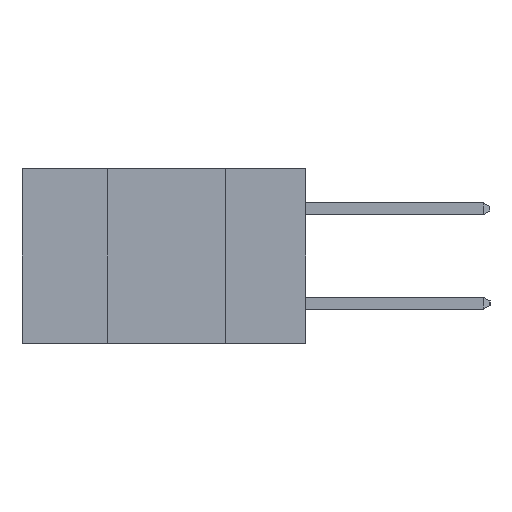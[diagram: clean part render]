
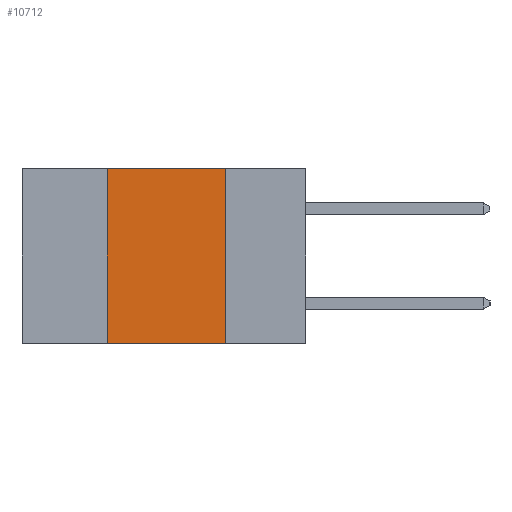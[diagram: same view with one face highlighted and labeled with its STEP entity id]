
A CAD part, left-side view. The second image highlights one B-rep face of the part: STEP entity #10712.
In plain terms, the highlighted planar face has unit normal (-1, 0, 0).
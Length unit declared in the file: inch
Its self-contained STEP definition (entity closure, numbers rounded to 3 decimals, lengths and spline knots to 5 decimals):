
#180 = VERTEX_POINT ( 'NONE', #7360 ) ;
#185 = LINE ( 'NONE', #12906, #5595 ) ;
#232 = DIRECTION ( 'NONE',  ( 0., 0., -1. ) ) ;
#284 = EDGE_CURVE ( 'NONE', #180, #655, #185, .T. ) ;
#655 = VERTEX_POINT ( 'NONE', #11268 ) ;
#1054 = ORIENTED_EDGE ( 'NONE', *, *, #6741, .F. ) ;
#1113 = DIRECTION ( 'NONE',  ( 1., 0., 0. ) ) ;
#2230 = CARTESIAN_POINT ( 'NONE',  ( 0., 0.42, 0. ) ) ;
#2700 = ORIENTED_EDGE ( 'NONE', *, *, #12487, .F. ) ;
#3275 = FACE_OUTER_BOUND ( 'NONE', #8496, .T. ) ;
#3808 = VECTOR ( 'NONE', #12885, 39.37008 ) ;
#4517 = AXIS2_PLACEMENT_3D ( 'NONE', #13466, #1113, #8454 ) ;
#4880 = VERTEX_POINT ( 'NONE', #4964 ) ;
#4964 = CARTESIAN_POINT ( 'NONE',  ( 0., 0.42, -0.37 ) ) ;
#5595 = VECTOR ( 'NONE', #232, 39.37008 ) ;
#5681 = LINE ( 'NONE', #6523, #10873 ) ;
#6390 = PLANE ( 'NONE',  #4517 ) ;
#6523 = CARTESIAN_POINT ( 'NONE',  ( 0., 0.6, 0. ) ) ;
#6741 = EDGE_CURVE ( 'NONE', #4880, #7665, #12022, .T. ) ;
#7097 = LINE ( 'NONE', #9097, #9221 ) ;
#7360 = CARTESIAN_POINT ( 'NONE',  ( 0., 0.17, 0. ) ) ;
#7466 = ORIENTED_EDGE ( 'NONE', *, *, #284, .F. ) ;
#7665 = VERTEX_POINT ( 'NONE', #2230 ) ;
#8355 = EDGE_CURVE ( 'NONE', #4880, #655, #7097, .T. ) ;
#8454 = DIRECTION ( 'NONE',  ( 0., 0., -1. ) ) ;
#8496 = EDGE_LOOP ( 'NONE', ( #7466, #2700, #1054, #11999 ) ) ;
#8598 = DIRECTION ( 'NONE',  ( 0., -1., 0. ) ) ;
#9061 = DIRECTION ( 'NONE',  ( 0., -1., 0. ) ) ;
#9097 = CARTESIAN_POINT ( 'NONE',  ( 0., 0.6, -0.37 ) ) ;
#9221 = VECTOR ( 'NONE', #9061, 39.37008 ) ;
#10712 = ADVANCED_FACE ( 'NONE', ( #3275 ), #6390, .F. ) ;
#10873 = VECTOR ( 'NONE', #8598, 39.37008 ) ;
#11268 = CARTESIAN_POINT ( 'NONE',  ( 0., 0.17, -0.37 ) ) ;
#11999 = ORIENTED_EDGE ( 'NONE', *, *, #8355, .T. ) ;
#12022 = LINE ( 'NONE', #12812, #3808 ) ;
#12487 = EDGE_CURVE ( 'NONE', #7665, #180, #5681, .T. ) ;
#12812 = CARTESIAN_POINT ( 'NONE',  ( 0., 0.42, -0.37 ) ) ;
#12885 = DIRECTION ( 'NONE',  ( 0., 0., 1. ) ) ;
#12906 = CARTESIAN_POINT ( 'NONE',  ( 0., 0.17, -0.37 ) ) ;
#13466 = CARTESIAN_POINT ( 'NONE',  ( 0., 0.6, 0. ) ) ;
